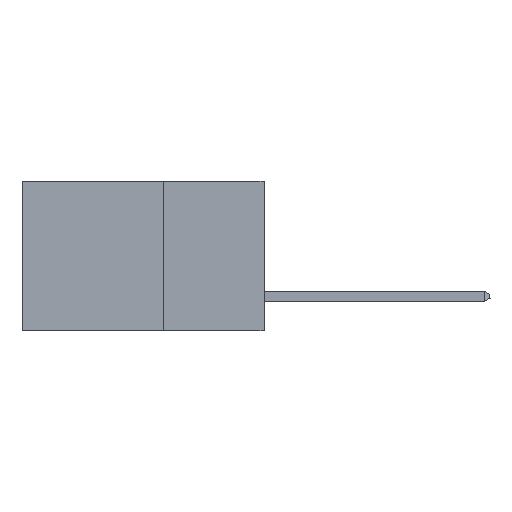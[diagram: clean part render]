
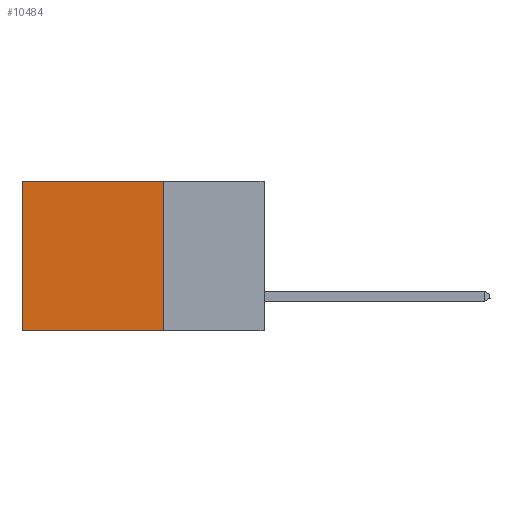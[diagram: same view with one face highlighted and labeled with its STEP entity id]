
A CAD part, left-side view. The second image highlights one B-rep face of the part: STEP entity #10484.
In plain terms, the highlighted planar face has unit normal (-1, 0, 0).
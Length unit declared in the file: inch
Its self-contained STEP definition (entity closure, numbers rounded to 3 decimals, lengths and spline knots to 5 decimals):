
#129 = VERTEX_POINT ( 'NONE', #2005 ) ;
#735 = VECTOR ( 'NONE', #1531, 39.37008 ) ;
#1371 = EDGE_LOOP ( 'NONE', ( #11443, #5707, #14884, #3475 ) ) ;
#1436 = DIRECTION ( 'NONE',  ( 0., 0., -1. ) ) ;
#1531 = DIRECTION ( 'NONE',  ( 0., 1., 0. ) ) ;
#1732 = DIRECTION ( 'NONE',  ( 0., 0., -1. ) ) ;
#1792 = CARTESIAN_POINT ( 'NONE',  ( 0.298, 0.25, 0. ) ) ;
#2005 = CARTESIAN_POINT ( 'NONE',  ( 0.298, 0.6, -0.37 ) ) ;
#3475 = ORIENTED_EDGE ( 'NONE', *, *, #6452, .T. ) ;
#4228 = VECTOR ( 'NONE', #14679, 39.37008 ) ;
#5031 = VERTEX_POINT ( 'NONE', #10613 ) ;
#5426 = CARTESIAN_POINT ( 'NONE',  ( 0.298, 0.25, 0. ) ) ;
#5509 = FACE_OUTER_BOUND ( 'NONE', #1371, .T. ) ;
#5561 = VECTOR ( 'NONE', #1732, 39.37008 ) ;
#5707 = ORIENTED_EDGE ( 'NONE', *, *, #15234, .F. ) ;
#5746 = PLANE ( 'NONE',  #10757 ) ;
#6262 = VERTEX_POINT ( 'NONE', #9023 ) ;
#6333 = CARTESIAN_POINT ( 'NONE',  ( 0.298, 0.6, 0. ) ) ;
#6452 = EDGE_CURVE ( 'NONE', #11199, #5031, #12404, .T. ) ;
#7020 = DIRECTION ( 'NONE',  ( 1., 0., 0. ) ) ;
#7675 = LINE ( 'NONE', #5426, #5561 ) ;
#8263 = DIRECTION ( 'NONE',  ( 0., 0., -1. ) ) ;
#8603 = VECTOR ( 'NONE', #1436, 39.37008 ) ;
#9023 = CARTESIAN_POINT ( 'NONE',  ( 0.298, 0.25, -0.37 ) ) ;
#9545 = EDGE_CURVE ( 'NONE', #11199, #6262, #7675, .T. ) ;
#10484 = ADVANCED_FACE ( 'NONE', ( #5509 ), #5746, .F. ) ;
#10613 = CARTESIAN_POINT ( 'NONE',  ( 0.298, 0.6, 0. ) ) ;
#10757 = AXIS2_PLACEMENT_3D ( 'NONE', #15605, #7020, #8263 ) ;
#10832 = CARTESIAN_POINT ( 'NONE',  ( 0.298, 0.25, 0. ) ) ;
#11064 = LINE ( 'NONE', #6333, #8603 ) ;
#11199 = VERTEX_POINT ( 'NONE', #10832 ) ;
#11443 = ORIENTED_EDGE ( 'NONE', *, *, #14182, .T. ) ;
#12404 = LINE ( 'NONE', #1792, #735 ) ;
#13408 = LINE ( 'NONE', #15646, #4228 ) ;
#14182 = EDGE_CURVE ( 'NONE', #5031, #129, #11064, .T. ) ;
#14679 = DIRECTION ( 'NONE',  ( 0., 1., 0. ) ) ;
#14884 = ORIENTED_EDGE ( 'NONE', *, *, #9545, .F. ) ;
#15234 = EDGE_CURVE ( 'NONE', #6262, #129, #13408, .T. ) ;
#15605 = CARTESIAN_POINT ( 'NONE',  ( 0.298, 0.25, 0. ) ) ;
#15646 = CARTESIAN_POINT ( 'NONE',  ( 0.298, 0.25, -0.37 ) ) ;
